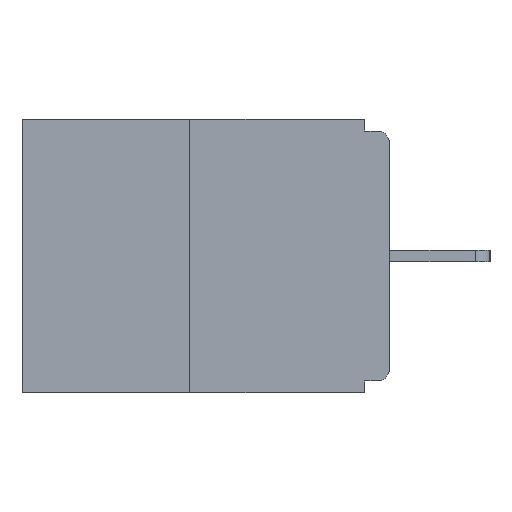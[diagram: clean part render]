
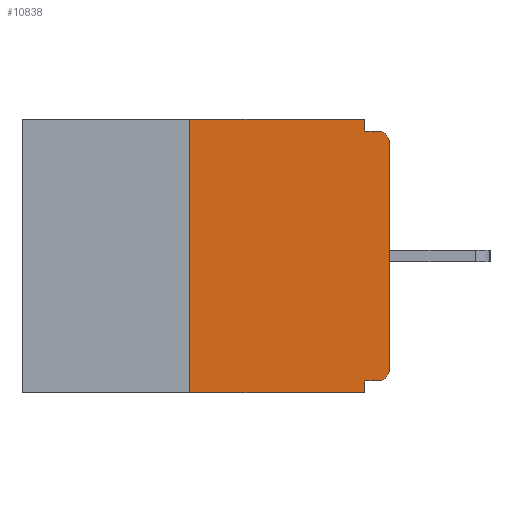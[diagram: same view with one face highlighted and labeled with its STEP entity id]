
A CAD part, left-side view. The second image highlights one B-rep face of the part: STEP entity #10838.
In plain terms, the highlighted planar face has unit normal (-1, 0, 0).
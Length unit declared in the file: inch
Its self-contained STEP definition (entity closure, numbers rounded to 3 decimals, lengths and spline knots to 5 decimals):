
#102 = EDGE_CURVE ( 'NONE', #8456, #1231, #12267, .T. ) ;
#745 = EDGE_LOOP ( 'NONE', ( #14957, #8503, #6122, #6168, #1830, #803, #3769, #13188, #13045, #3967 ) ) ;
#803 = ORIENTED_EDGE ( 'NONE', *, *, #11190, .T. ) ;
#916 = CARTESIAN_POINT ( 'NONE',  ( 0., 0., -0.015 ) ) ;
#1231 = VERTEX_POINT ( 'NONE', #8908 ) ;
#1580 = CARTESIAN_POINT ( 'NONE',  ( 0., 0., -0.328 ) ) ;
#1830 = ORIENTED_EDGE ( 'NONE', *, *, #12114, .F. ) ;
#1976 = VECTOR ( 'NONE', #8379, 39.37008 ) ;
#2192 = VECTOR ( 'NONE', #2356, 39.37008 ) ;
#2356 = DIRECTION ( 'NONE',  ( 0., 0., 1. ) ) ;
#2622 = FACE_OUTER_BOUND ( 'NONE', #745, .T. ) ;
#3476 = VECTOR ( 'NONE', #15164, 39.37008 ) ;
#3769 = ORIENTED_EDGE ( 'NONE', *, *, #16396, .T. ) ;
#3967 = ORIENTED_EDGE ( 'NONE', *, *, #4826, .F. ) ;
#4021 = EDGE_CURVE ( 'NONE', #10567, #14380, #9357, .T. ) ;
#4074 = CARTESIAN_POINT ( 'NONE',  ( 0., 0.015, -0.328 ) ) ;
#4826 = EDGE_CURVE ( 'NONE', #14380, #10521, #10813, .T. ) ;
#4924 = VERTEX_POINT ( 'NONE', #14093 ) ;
#5646 = VECTOR ( 'NONE', #16279, 39.37008 ) ;
#5676 = VECTOR ( 'NONE', #12549, 39.37008 ) ;
#6122 = ORIENTED_EDGE ( 'NONE', *, *, #102, .T. ) ;
#6168 = ORIENTED_EDGE ( 'NONE', *, *, #18088, .F. ) ;
#6463 = DIRECTION ( 'NONE',  ( 0., 0., -1. ) ) ;
#6702 = CARTESIAN_POINT ( 'NONE',  ( 0., 0.46, 0. ) ) ;
#6920 = DIRECTION ( 'NONE',  ( -1., 0., 0. ) ) ;
#7147 = DIRECTION ( 'NONE',  ( 0., 0., -1. ) ) ;
#7969 = CARTESIAN_POINT ( 'NONE',  ( 0., 0.031, 0. ) ) ;
#8319 = CARTESIAN_POINT ( 'NONE',  ( 0., 0.25, -0.343 ) ) ;
#8379 = DIRECTION ( 'NONE',  ( 0., 1., 0. ) ) ;
#8456 = VERTEX_POINT ( 'NONE', #8319 ) ;
#8503 = ORIENTED_EDGE ( 'NONE', *, *, #8874, .F. ) ;
#8572 = AXIS2_PLACEMENT_3D ( 'NONE', #15709, #14124, #7147 ) ;
#8652 = LINE ( 'NONE', #1580, #1976 ) ;
#8874 = EDGE_CURVE ( 'NONE', #8456, #10567, #14046, .T. ) ;
#8908 = CARTESIAN_POINT ( 'NONE',  ( 0., 0.031, -0.343 ) ) ;
#9357 = LINE ( 'NONE', #6702, #5676 ) ;
#9505 = AXIS2_PLACEMENT_3D ( 'NONE', #12403, #18148, #6463 ) ;
#9631 = CARTESIAN_POINT ( 'NONE',  ( 0., 0.46, -0.343 ) ) ;
#9694 = CARTESIAN_POINT ( 'NONE',  ( 0., 0.25, 0. ) ) ;
#9705 = VERTEX_POINT ( 'NONE', #4074 ) ;
#10521 = VERTEX_POINT ( 'NONE', #14217 ) ;
#10567 = VERTEX_POINT ( 'NONE', #9694 ) ;
#10640 = CARTESIAN_POINT ( 'NONE',  ( 0., 0.031, -0.343 ) ) ;
#10813 = LINE ( 'NONE', #7969, #14162 ) ;
#10838 = ADVANCED_FACE ( 'NONE', ( #2622 ), #14303, .F. ) ;
#11007 = VERTEX_POINT ( 'NONE', #14491 ) ;
#11120 = LINE ( 'NONE', #916, #3476 ) ;
#11165 = CARTESIAN_POINT ( 'NONE',  ( 0., 0.015, -0.313 ) ) ;
#11190 = EDGE_CURVE ( 'NONE', #9705, #11007, #17006, .T. ) ;
#11963 = CARTESIAN_POINT ( 'NONE',  ( 0., 0., 0. ) ) ;
#12114 = EDGE_CURVE ( 'NONE', #9705, #14284, #8652, .T. ) ;
#12240 = DIRECTION ( 'NONE',  ( 0., 0., 1. ) ) ;
#12267 = LINE ( 'NONE', #9631, #17602 ) ;
#12403 = CARTESIAN_POINT ( 'NONE',  ( 0., 0.015, -0.03 ) ) ;
#12549 = DIRECTION ( 'NONE',  ( 0., -1., 0. ) ) ;
#12659 = DIRECTION ( 'NONE',  ( 0., 0., -1. ) ) ;
#13045 = ORIENTED_EDGE ( 'NONE', *, *, #13278, .F. ) ;
#13188 = ORIENTED_EDGE ( 'NONE', *, *, #13748, .T. ) ;
#13261 = CARTESIAN_POINT ( 'NONE',  ( 0., 0., -0.03 ) ) ;
#13278 = EDGE_CURVE ( 'NONE', #10521, #4924, #11120, .T. ) ;
#13284 = LINE ( 'NONE', #11963, #14076 ) ;
#13451 = LINE ( 'NONE', #10640, #5646 ) ;
#13748 = EDGE_CURVE ( 'NONE', #16869, #4924, #17619, .T. ) ;
#14046 = LINE ( 'NONE', #18184, #2192 ) ;
#14076 = VECTOR ( 'NONE', #12240, 39.37008 ) ;
#14093 = CARTESIAN_POINT ( 'NONE',  ( 0., 0.015, -0.015 ) ) ;
#14124 = DIRECTION ( 'NONE',  ( 1., 0., 0. ) ) ;
#14162 = VECTOR ( 'NONE', #14940, 39.37008 ) ;
#14217 = CARTESIAN_POINT ( 'NONE',  ( 0., 0.031, -0.015 ) ) ;
#14284 = VERTEX_POINT ( 'NONE', #15766 ) ;
#14303 = PLANE ( 'NONE',  #8572 ) ;
#14380 = VERTEX_POINT ( 'NONE', #17729 ) ;
#14491 = CARTESIAN_POINT ( 'NONE',  ( 0., 0., -0.313 ) ) ;
#14940 = DIRECTION ( 'NONE',  ( 0., 0., -1. ) ) ;
#14957 = ORIENTED_EDGE ( 'NONE', *, *, #4021, .F. ) ;
#15164 = DIRECTION ( 'NONE',  ( 0., -1., 0. ) ) ;
#15709 = CARTESIAN_POINT ( 'NONE',  ( 0., 0.46, 0. ) ) ;
#15766 = CARTESIAN_POINT ( 'NONE',  ( 0., 0.031, -0.328 ) ) ;
#16279 = DIRECTION ( 'NONE',  ( 0., 0., -1. ) ) ;
#16396 = EDGE_CURVE ( 'NONE', #11007, #16869, #13284, .T. ) ;
#16869 = VERTEX_POINT ( 'NONE', #13261 ) ;
#16876 = DIRECTION ( 'NONE',  ( 0., -1., 0. ) ) ;
#17006 = CIRCLE ( 'NONE', #17296, 0.015 ) ;
#17296 = AXIS2_PLACEMENT_3D ( 'NONE', #11165, #6920, #12659 ) ;
#17602 = VECTOR ( 'NONE', #16876, 39.37008 ) ;
#17619 = CIRCLE ( 'NONE', #9505, 0.015 ) ;
#17729 = CARTESIAN_POINT ( 'NONE',  ( 0., 0.031, 0. ) ) ;
#18088 = EDGE_CURVE ( 'NONE', #14284, #1231, #13451, .T. ) ;
#18148 = DIRECTION ( 'NONE',  ( -1., 0., 0. ) ) ;
#18184 = CARTESIAN_POINT ( 'NONE',  ( 0., 0.25, 0. ) ) ;
